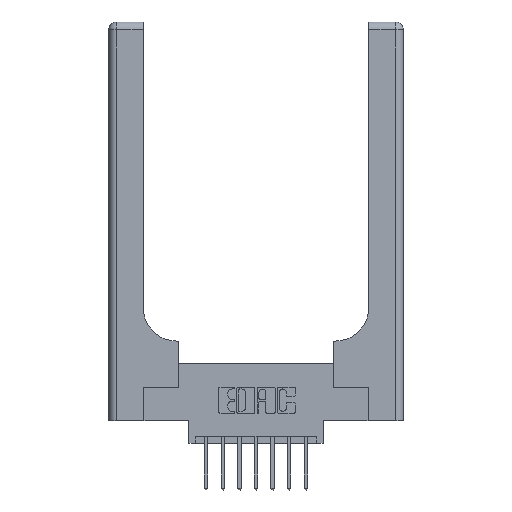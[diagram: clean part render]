
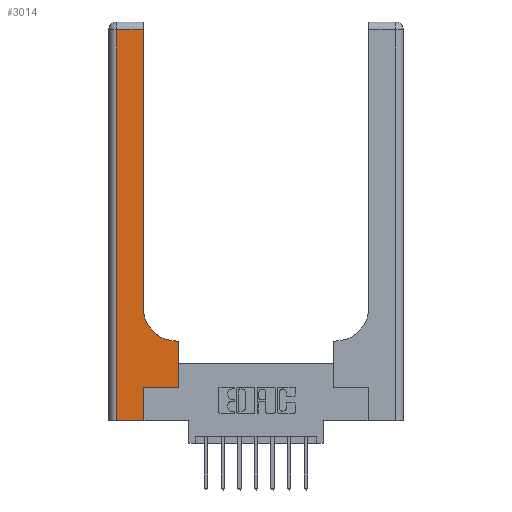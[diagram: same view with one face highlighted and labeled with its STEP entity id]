
A CAD part, top view. The second image highlights one B-rep face of the part: STEP entity #3014.
In plain terms, the highlighted planar face has unit normal (0, 0, 1).
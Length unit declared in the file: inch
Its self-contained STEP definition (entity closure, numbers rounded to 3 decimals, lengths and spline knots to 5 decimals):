
#9 = DIRECTION ( 'NONE',  ( 0., 1., 0. ) ) ;
#99 = VERTEX_POINT ( 'NONE', #1392 ) ;
#269 = EDGE_CURVE ( 'NONE', #6361, #12036, #11918, .T. ) ;
#645 = CARTESIAN_POINT ( 'NONE',  ( 0.26, 2.94, 0.37 ) ) ;
#671 = DIRECTION ( 'NONE',  ( 1., 0., 0. ) ) ;
#714 = CARTESIAN_POINT ( 'NONE',  ( 0.528, 0.6, 0.37 ) ) ;
#853 = EDGE_CURVE ( 'NONE', #8184, #13187, #13534, .T. ) ;
#886 = CARTESIAN_POINT ( 'NONE',  ( 0.26, 3., 0.37 ) ) ;
#918 = EDGE_LOOP ( 'NONE', ( #4516, #11582, #3608, #10039, #10232, #12367, #7286, #2409, #14471 ) ) ;
#1102 = DIRECTION ( 'NONE',  ( 0., 0., -1. ) ) ;
#1119 = LINE ( 'NONE', #13193, #7228 ) ;
#1392 = CARTESIAN_POINT ( 'NONE',  ( 0.265, 0., 0.37 ) ) ;
#1464 = EDGE_CURVE ( 'NONE', #12036, #8184, #1873, .T. ) ;
#1518 = VECTOR ( 'NONE', #13089, 39.37008 ) ;
#1873 = CIRCLE ( 'NONE', #13018, 0.25 ) ;
#1970 = DIRECTION ( 'NONE',  ( 0., 0., -1. ) ) ;
#2169 = LINE ( 'NONE', #7550, #13814 ) ;
#2409 = ORIENTED_EDGE ( 'NONE', *, *, #269, .T. ) ;
#2900 = EDGE_CURVE ( 'NONE', #8387, #11909, #2169, .T. ) ;
#3014 = ADVANCED_FACE ( 'NONE', ( #6844 ), #8772, .F. ) ;
#3181 = LINE ( 'NONE', #3459, #11826 ) ;
#3459 = CARTESIAN_POINT ( 'NONE',  ( 0.265, 0., 0.37 ) ) ;
#3608 = ORIENTED_EDGE ( 'NONE', *, *, #3883, .T. ) ;
#3795 = VECTOR ( 'NONE', #9313, 39.37008 ) ;
#3883 = EDGE_CURVE ( 'NONE', #10296, #4328, #11894, .T. ) ;
#4328 = VERTEX_POINT ( 'NONE', #7290 ) ;
#4516 = ORIENTED_EDGE ( 'NONE', *, *, #853, .T. ) ;
#4619 = DIRECTION ( 'NONE',  ( 0., 1., 0. ) ) ;
#6361 = VERTEX_POINT ( 'NONE', #714 ) ;
#6806 = LINE ( 'NONE', #13754, #3795 ) ;
#6844 = FACE_OUTER_BOUND ( 'NONE', #918, .T. ) ;
#7159 = EDGE_CURVE ( 'NONE', #99, #8387, #3181, .T. ) ;
#7228 = VECTOR ( 'NONE', #14287, 39.37008 ) ;
#7286 = ORIENTED_EDGE ( 'NONE', *, *, #12730, .T. ) ;
#7290 = CARTESIAN_POINT ( 'NONE',  ( 0.06, 0., 0.37 ) ) ;
#7454 = DIRECTION ( 'NONE',  ( 0., -1., 0. ) ) ;
#7550 = CARTESIAN_POINT ( 'NONE',  ( 0.265, 0.25, 0.37 ) ) ;
#7955 = CARTESIAN_POINT ( 'NONE',  ( 0.51, 0.85, 0.37 ) ) ;
#8184 = VERTEX_POINT ( 'NONE', #8738 ) ;
#8309 = EDGE_CURVE ( 'NONE', #4328, #99, #6806, .T. ) ;
#8387 = VERTEX_POINT ( 'NONE', #8403 ) ;
#8403 = CARTESIAN_POINT ( 'NONE',  ( 0.265, 0.25, 0.37 ) ) ;
#8732 = CARTESIAN_POINT ( 'NONE',  ( 0., 3., 0.37 ) ) ;
#8738 = CARTESIAN_POINT ( 'NONE',  ( 0.26, 0.85, 0.37 ) ) ;
#8772 = PLANE ( 'NONE',  #14577 ) ;
#9030 = DIRECTION ( 'NONE',  ( -1., 0., 0. ) ) ;
#9059 = DIRECTION ( 'NONE',  ( 1., 0., 0. ) ) ;
#9132 = CARTESIAN_POINT ( 'NONE',  ( 0.26, 0.6, 0.37 ) ) ;
#9313 = DIRECTION ( 'NONE',  ( 1., 0., 0. ) ) ;
#9539 = CARTESIAN_POINT ( 'NONE',  ( 0.528, 0.25, 0.37 ) ) ;
#9920 = DIRECTION ( 'NONE',  ( -1., 0., 0. ) ) ;
#10039 = ORIENTED_EDGE ( 'NONE', *, *, #8309, .T. ) ;
#10232 = ORIENTED_EDGE ( 'NONE', *, *, #7159, .T. ) ;
#10296 = VERTEX_POINT ( 'NONE', #10664 ) ;
#10352 = VECTOR ( 'NONE', #9030, 39.37008 ) ;
#10562 = LINE ( 'NONE', #10838, #1518 ) ;
#10577 = VECTOR ( 'NONE', #9, 39.37008 ) ;
#10664 = CARTESIAN_POINT ( 'NONE',  ( 0.06, 2.94, 0.37 ) ) ;
#10838 = CARTESIAN_POINT ( 'NONE',  ( 0.528, 0.25, 0.37 ) ) ;
#11541 = VECTOR ( 'NONE', #7454, 39.37008 ) ;
#11582 = ORIENTED_EDGE ( 'NONE', *, *, #13732, .T. ) ;
#11826 = VECTOR ( 'NONE', #4619, 39.37008 ) ;
#11894 = LINE ( 'NONE', #14090, #11541 ) ;
#11909 = VERTEX_POINT ( 'NONE', #9539 ) ;
#11918 = LINE ( 'NONE', #9132, #10352 ) ;
#12036 = VERTEX_POINT ( 'NONE', #13105 ) ;
#12367 = ORIENTED_EDGE ( 'NONE', *, *, #2900, .T. ) ;
#12730 = EDGE_CURVE ( 'NONE', #11909, #6361, #10562, .T. ) ;
#13018 = AXIS2_PLACEMENT_3D ( 'NONE', #7955, #1102, #9059 ) ;
#13089 = DIRECTION ( 'NONE',  ( 0., 1., 0. ) ) ;
#13105 = CARTESIAN_POINT ( 'NONE',  ( 0.51, 0.6, 0.37 ) ) ;
#13187 = VERTEX_POINT ( 'NONE', #645 ) ;
#13193 = CARTESIAN_POINT ( 'NONE',  ( 0., 2.94, 0.37 ) ) ;
#13534 = LINE ( 'NONE', #886, #10577 ) ;
#13732 = EDGE_CURVE ( 'NONE', #13187, #10296, #1119, .T. ) ;
#13754 = CARTESIAN_POINT ( 'NONE',  ( 0., 0., 0.37 ) ) ;
#13814 = VECTOR ( 'NONE', #671, 39.37008 ) ;
#14090 = CARTESIAN_POINT ( 'NONE',  ( 0.06, 3., 0.37 ) ) ;
#14287 = DIRECTION ( 'NONE',  ( -1., 0., 0. ) ) ;
#14471 = ORIENTED_EDGE ( 'NONE', *, *, #1464, .T. ) ;
#14577 = AXIS2_PLACEMENT_3D ( 'NONE', #8732, #1970, #9920 ) ;
